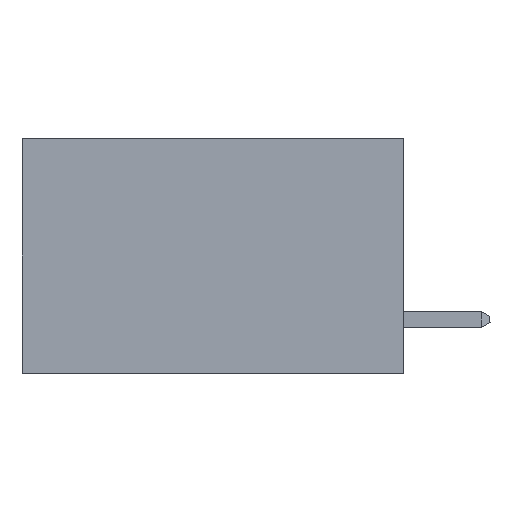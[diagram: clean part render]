
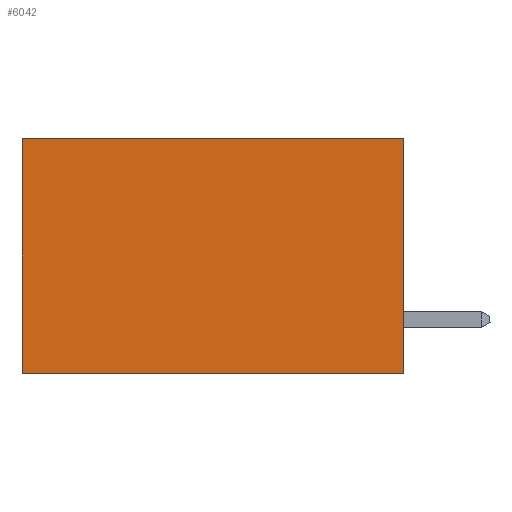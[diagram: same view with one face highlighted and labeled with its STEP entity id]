
A CAD part, left-side view. The second image highlights one B-rep face of the part: STEP entity #6042.
In plain terms, the highlighted planar face has unit normal (-1, 0, 0).
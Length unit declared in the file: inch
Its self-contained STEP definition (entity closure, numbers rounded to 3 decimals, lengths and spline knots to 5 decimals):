
#620 = EDGE_CURVE ( 'NONE', #5191, #7155, #6566, .T. ) ;
#1607 = VECTOR ( 'NONE', #3754, 39.37008 ) ;
#1781 = CARTESIAN_POINT ( 'NONE',  ( 0.2875, 0.6, 0. ) ) ;
#1833 = DIRECTION ( 'NONE',  ( 0., 1., 0. ) ) ;
#1897 = VECTOR ( 'NONE', #2541, 39.37008 ) ;
#2022 = CARTESIAN_POINT ( 'NONE',  ( 0.2875, 0., 0. ) ) ;
#2085 = EDGE_CURVE ( 'NONE', #3681, #2713, #7530, .T. ) ;
#2541 = DIRECTION ( 'NONE',  ( 0., 1., 0. ) ) ;
#2713 = VERTEX_POINT ( 'NONE', #4044 ) ;
#3054 = CARTESIAN_POINT ( 'NONE',  ( 0.2875, 0.6, -0.37 ) ) ;
#3681 = VERTEX_POINT ( 'NONE', #7097 ) ;
#3754 = DIRECTION ( 'NONE',  ( 0., 0., -1. ) ) ;
#4044 = CARTESIAN_POINT ( 'NONE',  ( 0.2875, 0., -0.37 ) ) ;
#4175 = EDGE_CURVE ( 'NONE', #2713, #7155, #6944, .T. ) ;
#4540 = DIRECTION ( 'NONE',  ( 0., 0., -1. ) ) ;
#5118 = VECTOR ( 'NONE', #4540, 39.37008 ) ;
#5120 = EDGE_LOOP ( 'NONE', ( #8971, #5196, #7072, #8477 ) ) ;
#5191 = VERTEX_POINT ( 'NONE', #7815 ) ;
#5196 = ORIENTED_EDGE ( 'NONE', *, *, #4175, .F. ) ;
#5919 = CARTESIAN_POINT ( 'NONE',  ( 0.2875, 0., 0. ) ) ;
#6042 = ADVANCED_FACE ( 'NONE', ( #7571 ), #7606, .F. ) ;
#6371 = VECTOR ( 'NONE', #1833, 39.37008 ) ;
#6566 = LINE ( 'NONE', #1781, #5118 ) ;
#6598 = CARTESIAN_POINT ( 'NONE',  ( 0.2875, 0., 0. ) ) ;
#6845 = CARTESIAN_POINT ( 'NONE',  ( 0.2875, 0., -0.37 ) ) ;
#6944 = LINE ( 'NONE', #6845, #6371 ) ;
#7072 = ORIENTED_EDGE ( 'NONE', *, *, #2085, .F. ) ;
#7097 = CARTESIAN_POINT ( 'NONE',  ( 0.2875, 0., 0. ) ) ;
#7155 = VERTEX_POINT ( 'NONE', #3054 ) ;
#7530 = LINE ( 'NONE', #6598, #1607 ) ;
#7571 = FACE_OUTER_BOUND ( 'NONE', #5120, .T. ) ;
#7606 = PLANE ( 'NONE',  #8336 ) ;
#7698 = DIRECTION ( 'NONE',  ( 0., 0., -1. ) ) ;
#7815 = CARTESIAN_POINT ( 'NONE',  ( 0.2875, 0.6, 0. ) ) ;
#8168 = LINE ( 'NONE', #5919, #1897 ) ;
#8336 = AXIS2_PLACEMENT_3D ( 'NONE', #2022, #9001, #7698 ) ;
#8477 = ORIENTED_EDGE ( 'NONE', *, *, #8733, .T. ) ;
#8733 = EDGE_CURVE ( 'NONE', #3681, #5191, #8168, .T. ) ;
#8971 = ORIENTED_EDGE ( 'NONE', *, *, #620, .T. ) ;
#9001 = DIRECTION ( 'NONE',  ( 1., 0., 0. ) ) ;
